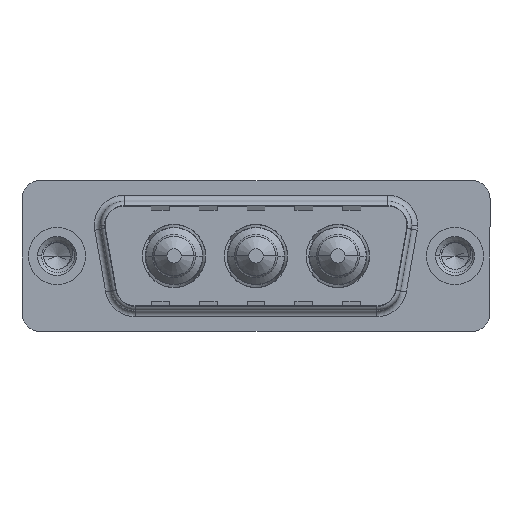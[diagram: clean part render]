
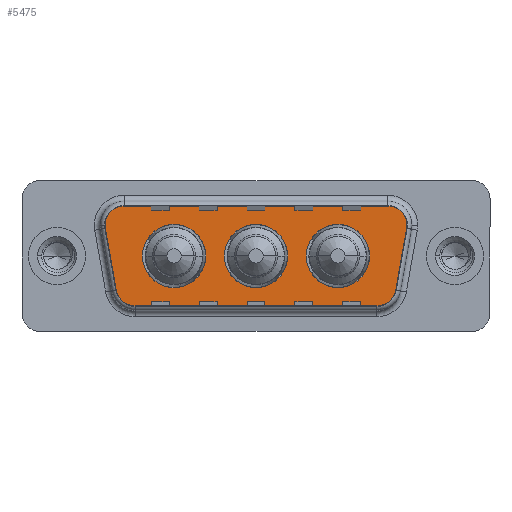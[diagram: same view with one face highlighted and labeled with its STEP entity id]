
A CAD part, top view. The second image highlights one B-rep face of the part: STEP entity #5475.
In plain terms, the highlighted planar face has unit normal (0, 0, 1).
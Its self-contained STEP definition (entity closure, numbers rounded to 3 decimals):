
#5 = CIRCLE ( 'NONE', #12388, 2. ) ;
#471 = EDGE_CURVE ( 'NONE', #9142, #11289, #6343, .T. ) ;
#512 = CARTESIAN_POINT ( 'NONE',  ( 4.464, -3.247, 0. ) ) ;
#523 = ORIENTED_EDGE ( 'NONE', *, *, #7638, .F. ) ;
#650 = AXIS2_PLACEMENT_3D ( 'NONE', #11160, #11327, #11127 ) ;
#769 = EDGE_CURVE ( 'NONE', #11742, #9480, #8553, .T. ) ;
#838 = VERTEX_POINT ( 'NONE', #512 ) ;
#924 = VECTOR ( 'NONE', #10030, 1000. ) ;
#1178 = VERTEX_POINT ( 'NONE', #1614 ) ;
#1215 = DIRECTION ( 'NONE',  ( 0., 0., 1. ) ) ;
#1347 = CARTESIAN_POINT ( 'NONE',  ( 28.836, -3.247, 0. ) ) ;
#1434 = VERTEX_POINT ( 'NONE', #1878 ) ;
#1560 = LINE ( 'NONE', #2528, #9788 ) ;
#1614 = CARTESIAN_POINT ( 'NONE',  ( 27.889, 4.9, 0. ) ) ;
#1634 = DIRECTION ( 'NONE',  ( 0., 0., 1. ) ) ;
#1648 = ORIENTED_EDGE ( 'NONE', *, *, #7185, .T. ) ;
#1774 = CARTESIAN_POINT ( 'NONE',  ( 6.434, -4.9, 0. ) ) ;
#1878 = CARTESIAN_POINT ( 'NONE',  ( 5.411, 4.9, 0. ) ) ;
#1951 = CARTESIAN_POINT ( 'NONE',  ( 16.65, 0., 0. ) ) ;
#1955 = AXIS2_PLACEMENT_3D ( 'NONE', #9568, #8605, #8582 ) ;
#1957 = EDGE_LOOP ( 'NONE', ( #3231, #11476, #3411, #3951, #3291, #6669, #5685, #5262, #1648 ) ) ;
#1962 = DIRECTION ( 'NONE',  ( 1., 0., 0. ) ) ;
#2124 = CIRCLE ( 'NONE', #5753, 2. ) ;
#2127 = AXIS2_PLACEMENT_3D ( 'NONE', #4272, #11535, #5397 ) ;
#2140 = VERTEX_POINT ( 'NONE', #10641 ) ;
#2289 = DIRECTION ( 'NONE',  ( 0.174, 0.985, 0. ) ) ;
#2426 = DIRECTION ( 'NONE',  ( 0., 0., 1. ) ) ;
#2428 = CARTESIAN_POINT ( 'NONE',  ( 12.45, 0., 0. ) ) ;
#2528 = CARTESIAN_POINT ( 'NONE',  ( 5.411, 4.9, 0. ) ) ;
#2650 = EDGE_CURVE ( 'NONE', #9480, #11742, #3844, .T. ) ;
#2699 = AXIS2_PLACEMENT_3D ( 'NONE', #8879, #2426, #9885 ) ;
#2703 = ORIENTED_EDGE ( 'NONE', *, *, #10152, .F. ) ;
#2819 = VECTOR ( 'NONE', #7173, 1000. ) ;
#2969 = CARTESIAN_POINT ( 'NONE',  ( 26.15, 0., 0. ) ) ;
#3064 = DIRECTION ( 'NONE',  ( 1., 0., 0. ) ) ;
#3110 = CARTESIAN_POINT ( 'NONE',  ( 5.411, 2.9, 0. ) ) ;
#3142 = CARTESIAN_POINT ( 'NONE',  ( 7.15, 0., 0. ) ) ;
#3231 = ORIENTED_EDGE ( 'NONE', *, *, #471, .T. ) ;
#3291 = ORIENTED_EDGE ( 'NONE', *, *, #9873, .T. ) ;
#3358 = CIRCLE ( 'NONE', #9017, 2.65 ) ;
#3403 = CARTESIAN_POINT ( 'NONE',  ( 20.85, 0., 0. ) ) ;
#3405 = EDGE_CURVE ( 'NONE', #13139, #10203, #8822, .T. ) ;
#3411 = ORIENTED_EDGE ( 'NONE', *, *, #6660, .T. ) ;
#3588 = CIRCLE ( 'NONE', #2699, 2. ) ;
#3844 = CIRCLE ( 'NONE', #1955, 2.65 ) ;
#3868 = CARTESIAN_POINT ( 'NONE',  ( 29.889, 2.9, 0. ) ) ;
#3951 = ORIENTED_EDGE ( 'NONE', *, *, #8966, .T. ) ;
#4152 = AXIS2_PLACEMENT_3D ( 'NONE', #10824, #4644, #11857 ) ;
#4245 = DIRECTION ( 'NONE',  ( 1., 0., 0. ) ) ;
#4272 = CARTESIAN_POINT ( 'NONE',  ( 16.65, 0., 0. ) ) ;
#4392 = VERTEX_POINT ( 'NONE', #1774 ) ;
#4644 = DIRECTION ( 'NONE',  ( 0., 0., 1. ) ) ;
#4671 = FACE_OUTER_BOUND ( 'NONE', #1957, .T. ) ;
#5164 = DIRECTION ( 'NONE',  ( 0., 0., 1. ) ) ;
#5262 = ORIENTED_EDGE ( 'NONE', *, *, #11820, .T. ) ;
#5266 = DIRECTION ( 'NONE',  ( 0., 0., 1. ) ) ;
#5397 = DIRECTION ( 'NONE',  ( 1., 0., 0. ) ) ;
#5439 = LINE ( 'NONE', #13261, #2819 ) ;
#5475 = ADVANCED_FACE ( 'NONE', ( #7525, #5704, #10193, #4671 ), #12070, .T. ) ;
#5685 = ORIENTED_EDGE ( 'NONE', *, *, #8897, .T. ) ;
#5704 = FACE_BOUND ( 'NONE', #6678, .T. ) ;
#5753 = AXIS2_PLACEMENT_3D ( 'NONE', #11296, #5164, #12334 ) ;
#6036 = EDGE_LOOP ( 'NONE', ( #9292, #523 ) ) ;
#6178 = EDGE_LOOP ( 'NONE', ( #11672, #2703 ) ) ;
#6343 = CIRCLE ( 'NONE', #8486, 2. ) ;
#6660 = EDGE_CURVE ( 'NONE', #2140, #13545, #7497, .T. ) ;
#6669 = ORIENTED_EDGE ( 'NONE', *, *, #13729, .T. ) ;
#6678 = EDGE_LOOP ( 'NONE', ( #9003, #10139 ) ) ;
#6878 = CARTESIAN_POINT ( 'NONE',  ( 9.8, 0., 0. ) ) ;
#6937 = CIRCLE ( 'NONE', #2127, 2.65 ) ;
#7173 = DIRECTION ( 'NONE',  ( 0.174, -0.985, 0. ) ) ;
#7185 = EDGE_CURVE ( 'NONE', #4392, #9142, #9549, .T. ) ;
#7497 = CIRCLE ( 'NONE', #12157, 2. ) ;
#7525 = FACE_BOUND ( 'NONE', #6178, .T. ) ;
#7592 = EDGE_CURVE ( 'NONE', #11289, #2140, #10751, .T. ) ;
#7638 = EDGE_CURVE ( 'NONE', #10203, #13139, #9840, .T. ) ;
#7880 = VERTEX_POINT ( 'NONE', #9202 ) ;
#8005 = AXIS2_PLACEMENT_3D ( 'NONE', #6878, #5266, #11312 ) ;
#8028 = CARTESIAN_POINT ( 'NONE',  ( 6.434, -4.9, 0. ) ) ;
#8184 = CARTESIAN_POINT ( 'NONE',  ( 27.889, 2.9, 0. ) ) ;
#8404 = CARTESIAN_POINT ( 'NONE',  ( 26.866, -2.9, 0. ) ) ;
#8486 = AXIS2_PLACEMENT_3D ( 'NONE', #8404, #1215, #1962 ) ;
#8553 = CIRCLE ( 'NONE', #12993, 2.65 ) ;
#8569 = DIRECTION ( 'NONE',  ( 0., 0., 1. ) ) ;
#8582 = DIRECTION ( 'NONE',  ( 1., 0., 0. ) ) ;
#8605 = DIRECTION ( 'NONE',  ( 0., 0., 1. ) ) ;
#8822 = CIRCLE ( 'NONE', #8005, 2.65 ) ;
#8879 = CARTESIAN_POINT ( 'NONE',  ( 6.434, -2.9, 0. ) ) ;
#8897 = EDGE_CURVE ( 'NONE', #7880, #838, #5439, .T. ) ;
#8966 = EDGE_CURVE ( 'NONE', #13545, #1178, #2124, .T. ) ;
#9003 = ORIENTED_EDGE ( 'NONE', *, *, #2650, .F. ) ;
#9017 = AXIS2_PLACEMENT_3D ( 'NONE', #1951, #9464, #3064 ) ;
#9142 = VERTEX_POINT ( 'NONE', #12901 ) ;
#9200 = DIRECTION ( 'NONE',  ( -1., 0., 0. ) ) ;
#9202 = CARTESIAN_POINT ( 'NONE',  ( 3.441, 2.553, 0. ) ) ;
#9254 = DIRECTION ( 'NONE',  ( 1., 0., 0. ) ) ;
#9292 = ORIENTED_EDGE ( 'NONE', *, *, #3405, .F. ) ;
#9297 = VERTEX_POINT ( 'NONE', #10074 ) ;
#9464 = DIRECTION ( 'NONE',  ( 0., 0., 1. ) ) ;
#9480 = VERTEX_POINT ( 'NONE', #2969 ) ;
#9549 = LINE ( 'NONE', #8028, #924 ) ;
#9568 = CARTESIAN_POINT ( 'NONE',  ( 23.5, 0., 0. ) ) ;
#9765 = CARTESIAN_POINT ( 'NONE',  ( 29.859, 2.553, 0. ) ) ;
#9788 = VECTOR ( 'NONE', #11997, 1000. ) ;
#9840 = CIRCLE ( 'NONE', #4152, 2.65 ) ;
#9873 = EDGE_CURVE ( 'NONE', #1178, #1434, #1560, .T. ) ;
#9885 = DIRECTION ( 'NONE',  ( -1., 0., 0. ) ) ;
#10030 = DIRECTION ( 'NONE',  ( 1., 0., 0. ) ) ;
#10074 = CARTESIAN_POINT ( 'NONE',  ( 19.3, 0., 0. ) ) ;
#10139 = ORIENTED_EDGE ( 'NONE', *, *, #769, .F. ) ;
#10152 = EDGE_CURVE ( 'NONE', #13693, #9297, #6937, .T. ) ;
#10193 = FACE_BOUND ( 'NONE', #6036, .T. ) ;
#10203 = VERTEX_POINT ( 'NONE', #3142 ) ;
#10488 = DIRECTION ( 'NONE',  ( 0., 0., 1. ) ) ;
#10641 = CARTESIAN_POINT ( 'NONE',  ( 29.859, 2.553, 0. ) ) ;
#10751 = LINE ( 'NONE', #9765, #13196 ) ;
#10824 = CARTESIAN_POINT ( 'NONE',  ( 9.8, 0., 0. ) ) ;
#11127 = DIRECTION ( 'NONE',  ( 1., 0., 0. ) ) ;
#11160 = CARTESIAN_POINT ( 'NONE',  ( 26.866, -2.9, 0. ) ) ;
#11289 = VERTEX_POINT ( 'NONE', #1347 ) ;
#11296 = CARTESIAN_POINT ( 'NONE',  ( 27.889, 2.9, 0. ) ) ;
#11312 = DIRECTION ( 'NONE',  ( 1., 0., 0. ) ) ;
#11327 = DIRECTION ( 'NONE',  ( 0., 0., 1. ) ) ;
#11366 = CARTESIAN_POINT ( 'NONE',  ( 14., 0., 0. ) ) ;
#11476 = ORIENTED_EDGE ( 'NONE', *, *, #7592, .T. ) ;
#11535 = DIRECTION ( 'NONE',  ( 0., 0., 1. ) ) ;
#11652 = CARTESIAN_POINT ( 'NONE',  ( 23.5, 0., 0. ) ) ;
#11672 = ORIENTED_EDGE ( 'NONE', *, *, #13697, .F. ) ;
#11742 = VERTEX_POINT ( 'NONE', #3403 ) ;
#11820 = EDGE_CURVE ( 'NONE', #838, #4392, #3588, .T. ) ;
#11857 = DIRECTION ( 'NONE',  ( 1., 0., 0. ) ) ;
#11997 = DIRECTION ( 'NONE',  ( -1., 0., 0. ) ) ;
#12070 = PLANE ( 'NONE',  #650 ) ;
#12157 = AXIS2_PLACEMENT_3D ( 'NONE', #8184, #1634, #9200 ) ;
#12334 = DIRECTION ( 'NONE',  ( -1., 0., 0. ) ) ;
#12388 = AXIS2_PLACEMENT_3D ( 'NONE', #3110, #10488, #4245 ) ;
#12901 = CARTESIAN_POINT ( 'NONE',  ( 26.866, -4.9, 0. ) ) ;
#12993 = AXIS2_PLACEMENT_3D ( 'NONE', #11652, #8569, #9254 ) ;
#13139 = VERTEX_POINT ( 'NONE', #2428 ) ;
#13196 = VECTOR ( 'NONE', #2289, 1000. ) ;
#13261 = CARTESIAN_POINT ( 'NONE',  ( 3.441, 2.553, 0. ) ) ;
#13545 = VERTEX_POINT ( 'NONE', #3868 ) ;
#13693 = VERTEX_POINT ( 'NONE', #11366 ) ;
#13697 = EDGE_CURVE ( 'NONE', #9297, #13693, #3358, .T. ) ;
#13729 = EDGE_CURVE ( 'NONE', #1434, #7880, #5, .T. ) ;
